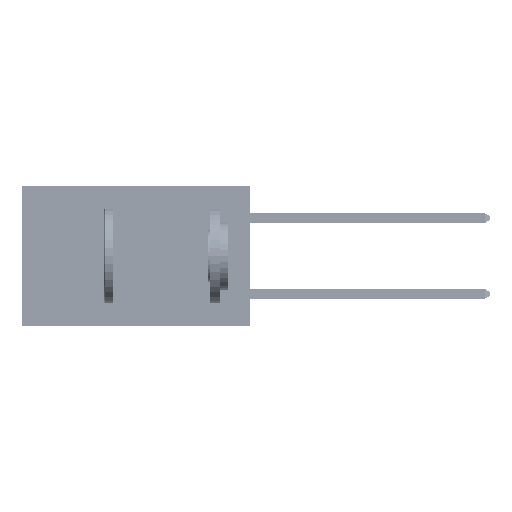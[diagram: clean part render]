
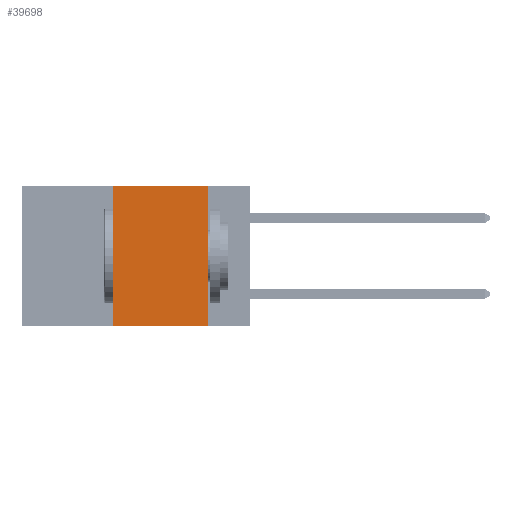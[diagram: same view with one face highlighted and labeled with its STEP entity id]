
A CAD part, left-side view. The second image highlights one B-rep face of the part: STEP entity #39698.
In plain terms, the highlighted planar face has unit normal (-1, 0, 0).
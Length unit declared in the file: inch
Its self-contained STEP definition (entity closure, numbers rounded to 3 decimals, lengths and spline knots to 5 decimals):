
#2831 = ORIENTED_EDGE ( 'NONE', *, *, #25045, .F. ) ;
#3750 = PLANE ( 'NONE',  #12680 ) ;
#6988 = CARTESIAN_POINT ( 'NONE',  ( 0., 0.11, 0. ) ) ;
#7441 = DIRECTION ( 'NONE',  ( 0., -1., 0. ) ) ;
#7572 = DIRECTION ( 'NONE',  ( 1., 0., 0. ) ) ;
#9228 = VECTOR ( 'NONE', #46785, 39.37008 ) ;
#9508 = CARTESIAN_POINT ( 'NONE',  ( 0., 0.36, -0.37 ) ) ;
#9835 = EDGE_CURVE ( 'NONE', #16915, #34602, #9855, .T. ) ;
#9855 = LINE ( 'NONE', #41206, #48618 ) ;
#10712 = EDGE_CURVE ( 'NONE', #34602, #44514, #12827, .T. ) ;
#11644 = VECTOR ( 'NONE', #23658, 39.37008 ) ;
#12680 = AXIS2_PLACEMENT_3D ( 'NONE', #18907, #7572, #34030 ) ;
#12827 = LINE ( 'NONE', #31045, #11644 ) ;
#14549 = CARTESIAN_POINT ( 'NONE',  ( 0., 0.36, 0. ) ) ;
#16762 = VECTOR ( 'NONE', #43018, 39.37008 ) ;
#16915 = VERTEX_POINT ( 'NONE', #14549 ) ;
#17970 = LINE ( 'NONE', #24257, #16762 ) ;
#18907 = CARTESIAN_POINT ( 'NONE',  ( 0., 0.6, 0. ) ) ;
#19699 = EDGE_CURVE ( 'NONE', #19743, #44514, #29392, .T. ) ;
#19743 = VERTEX_POINT ( 'NONE', #9508 ) ;
#23081 = ORIENTED_EDGE ( 'NONE', *, *, #19699, .T. ) ;
#23658 = DIRECTION ( 'NONE',  ( 0., 0., -1. ) ) ;
#24257 = CARTESIAN_POINT ( 'NONE',  ( 0., 0.36, 0. ) ) ;
#25045 = EDGE_CURVE ( 'NONE', #19743, #16915, #17970, .T. ) ;
#29392 = LINE ( 'NONE', #43066, #9228 ) ;
#30372 = EDGE_LOOP ( 'NONE', ( #34782, #48139, #2831, #23081 ) ) ;
#31045 = CARTESIAN_POINT ( 'NONE',  ( 0., 0.11, 0. ) ) ;
#34030 = DIRECTION ( 'NONE',  ( 0., 0., -1. ) ) ;
#34602 = VERTEX_POINT ( 'NONE', #6988 ) ;
#34782 = ORIENTED_EDGE ( 'NONE', *, *, #10712, .F. ) ;
#39698 = ADVANCED_FACE ( 'NONE', ( #39812 ), #3750, .F. ) ;
#39812 = FACE_OUTER_BOUND ( 'NONE', #30372, .T. ) ;
#41206 = CARTESIAN_POINT ( 'NONE',  ( 0., 0.6, 0. ) ) ;
#43018 = DIRECTION ( 'NONE',  ( 0., 0., 1. ) ) ;
#43066 = CARTESIAN_POINT ( 'NONE',  ( 0., 0.6, -0.37 ) ) ;
#43700 = CARTESIAN_POINT ( 'NONE',  ( 0., 0.11, -0.37 ) ) ;
#44514 = VERTEX_POINT ( 'NONE', #43700 ) ;
#46785 = DIRECTION ( 'NONE',  ( 0., -1., 0. ) ) ;
#48139 = ORIENTED_EDGE ( 'NONE', *, *, #9835, .F. ) ;
#48618 = VECTOR ( 'NONE', #7441, 39.37008 ) ;
